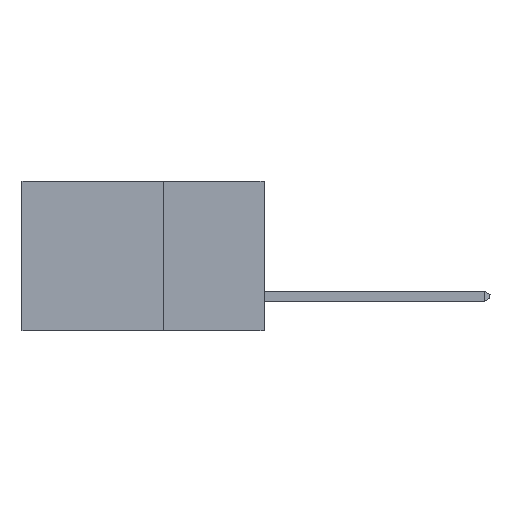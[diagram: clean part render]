
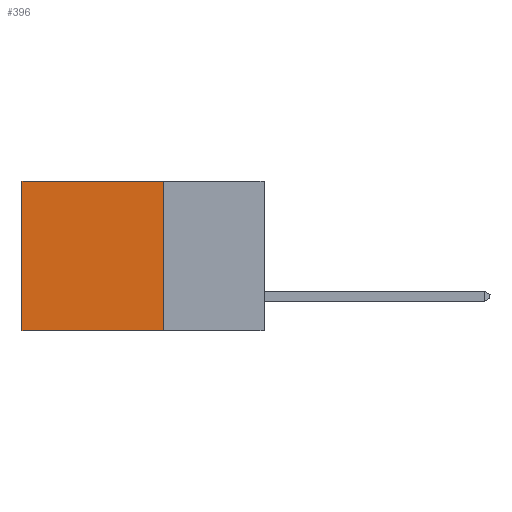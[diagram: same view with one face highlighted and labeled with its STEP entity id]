
A CAD part, left-side view. The second image highlights one B-rep face of the part: STEP entity #396.
In plain terms, the highlighted planar face has unit normal (-1, 0, 0).
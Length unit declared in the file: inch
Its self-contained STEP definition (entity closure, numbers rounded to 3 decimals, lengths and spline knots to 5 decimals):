
#199 = CARTESIAN_POINT ( 'NONE',  ( 0.298, 0.25, 0. ) ) ;
#396 = ADVANCED_FACE ( 'NONE', ( #7620 ), #9976, .F. ) ;
#580 = EDGE_LOOP ( 'NONE', ( #743, #6515, #8424, #8345 ) ) ;
#743 = ORIENTED_EDGE ( 'NONE', *, *, #2181, .T. ) ;
#1210 = CARTESIAN_POINT ( 'NONE',  ( 0.298, 0.25, 0. ) ) ;
#1361 = CARTESIAN_POINT ( 'NONE',  ( 0.298, 0.25, -0.37 ) ) ;
#1364 = VECTOR ( 'NONE', #13150, 39.37008 ) ;
#1426 = LINE ( 'NONE', #6017, #1591 ) ;
#1591 = VECTOR ( 'NONE', #1685, 39.37008 ) ;
#1681 = CARTESIAN_POINT ( 'NONE',  ( 0.298, 0.6, -0.37 ) ) ;
#1685 = DIRECTION ( 'NONE',  ( 0., 0., -1. ) ) ;
#1794 = CARTESIAN_POINT ( 'NONE',  ( 0.298, 0.6, 0. ) ) ;
#1896 = VECTOR ( 'NONE', #6326, 39.37008 ) ;
#2181 = EDGE_CURVE ( 'NONE', #9288, #8256, #1426, .T. ) ;
#3089 = CARTESIAN_POINT ( 'NONE',  ( 0.298, 0.25, 0. ) ) ;
#3133 = DIRECTION ( 'NONE',  ( 0., 1., 0. ) ) ;
#4014 = EDGE_CURVE ( 'NONE', #9323, #10577, #12218, .T. ) ;
#4797 = EDGE_CURVE ( 'NONE', #9323, #9288, #8330, .T. ) ;
#6017 = CARTESIAN_POINT ( 'NONE',  ( 0.298, 0.6, 0. ) ) ;
#6326 = DIRECTION ( 'NONE',  ( 0., 1., 0. ) ) ;
#6515 = ORIENTED_EDGE ( 'NONE', *, *, #6642, .F. ) ;
#6642 = EDGE_CURVE ( 'NONE', #10577, #8256, #11212, .T. ) ;
#7620 = FACE_OUTER_BOUND ( 'NONE', #580, .T. ) ;
#7966 = DIRECTION ( 'NONE',  ( 0., 0., -1. ) ) ;
#8256 = VERTEX_POINT ( 'NONE', #1681 ) ;
#8330 = LINE ( 'NONE', #3089, #11504 ) ;
#8345 = ORIENTED_EDGE ( 'NONE', *, *, #4797, .T. ) ;
#8424 = ORIENTED_EDGE ( 'NONE', *, *, #4014, .F. ) ;
#8896 = DIRECTION ( 'NONE',  ( 1., 0., 0. ) ) ;
#9181 = CARTESIAN_POINT ( 'NONE',  ( 0.298, 0.25, -0.37 ) ) ;
#9288 = VERTEX_POINT ( 'NONE', #1794 ) ;
#9323 = VERTEX_POINT ( 'NONE', #10502 ) ;
#9976 = PLANE ( 'NONE',  #13840 ) ;
#10502 = CARTESIAN_POINT ( 'NONE',  ( 0.298, 0.25, 0. ) ) ;
#10577 = VERTEX_POINT ( 'NONE', #1361 ) ;
#11212 = LINE ( 'NONE', #9181, #1896 ) ;
#11504 = VECTOR ( 'NONE', #3133, 39.37008 ) ;
#12218 = LINE ( 'NONE', #1210, #1364 ) ;
#13150 = DIRECTION ( 'NONE',  ( 0., 0., -1. ) ) ;
#13840 = AXIS2_PLACEMENT_3D ( 'NONE', #199, #8896, #7966 ) ;
